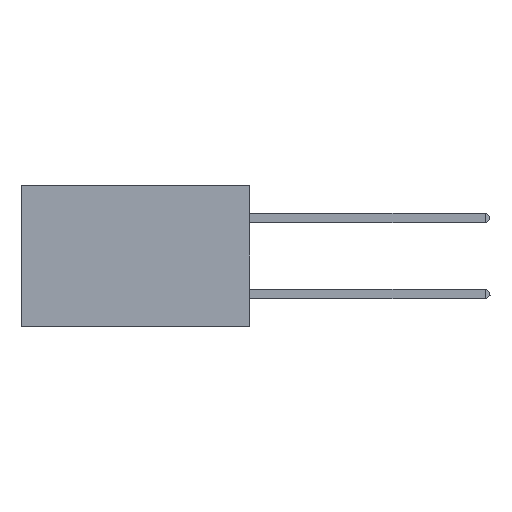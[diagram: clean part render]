
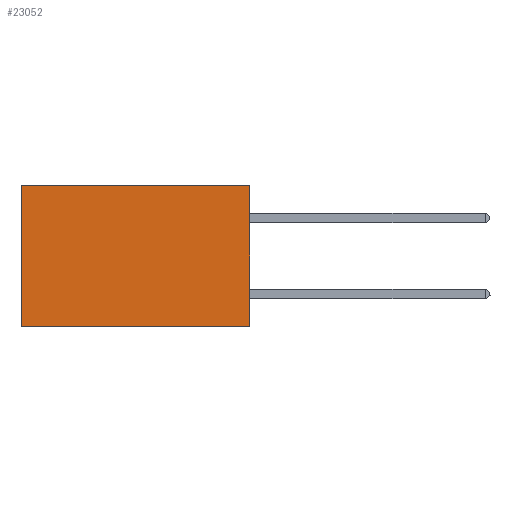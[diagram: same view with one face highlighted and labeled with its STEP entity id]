
A CAD part, left-side view. The second image highlights one B-rep face of the part: STEP entity #23052.
In plain terms, the highlighted planar face has unit normal (-1, 0, 0).
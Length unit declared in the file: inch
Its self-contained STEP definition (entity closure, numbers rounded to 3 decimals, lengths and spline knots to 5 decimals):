
#237 = FACE_OUTER_BOUND ( 'NONE', #17870, .T. ) ;
#645 = CARTESIAN_POINT ( 'NONE',  ( 0.2875, 0., 0. ) ) ;
#1793 = EDGE_CURVE ( 'NONE', #4694, #19247, #15864, .T. ) ;
#3028 = DIRECTION ( 'NONE',  ( 0., 0., -1. ) ) ;
#3229 = DIRECTION ( 'NONE',  ( 0., 0., -1. ) ) ;
#4694 = VERTEX_POINT ( 'NONE', #20214 ) ;
#5018 = EDGE_CURVE ( 'NONE', #10851, #4694, #14212, .T. ) ;
#5199 = DIRECTION ( 'NONE',  ( 0., 1., 0. ) ) ;
#7145 = EDGE_CURVE ( 'NONE', #10851, #10765, #13715, .T. ) ;
#8940 = DIRECTION ( 'NONE',  ( 0., 1., 0. ) ) ;
#9020 = ORIENTED_EDGE ( 'NONE', *, *, #13506, .F. ) ;
#9150 = ORIENTED_EDGE ( 'NONE', *, *, #7145, .F. ) ;
#10765 = VERTEX_POINT ( 'NONE', #15515 ) ;
#10851 = VERTEX_POINT ( 'NONE', #16892 ) ;
#13084 = CARTESIAN_POINT ( 'NONE',  ( 0.2875, 0., -0.37 ) ) ;
#13506 = EDGE_CURVE ( 'NONE', #10765, #19247, #14063, .T. ) ;
#13715 = LINE ( 'NONE', #645, #14093 ) ;
#14063 = LINE ( 'NONE', #13084, #25969 ) ;
#14093 = VECTOR ( 'NONE', #3028, 39.37008 ) ;
#14212 = LINE ( 'NONE', #28877, #22821 ) ;
#14662 = CARTESIAN_POINT ( 'NONE',  ( 0.2875, 0., 0. ) ) ;
#15515 = CARTESIAN_POINT ( 'NONE',  ( 0.2875, 0., -0.37 ) ) ;
#15864 = LINE ( 'NONE', #17469, #30058 ) ;
#16892 = CARTESIAN_POINT ( 'NONE',  ( 0.2875, 0., 0. ) ) ;
#17469 = CARTESIAN_POINT ( 'NONE',  ( 0.2875, 0.6, 0. ) ) ;
#17870 = EDGE_LOOP ( 'NONE', ( #21938, #9020, #9150, #18020 ) ) ;
#18020 = ORIENTED_EDGE ( 'NONE', *, *, #5018, .T. ) ;
#19247 = VERTEX_POINT ( 'NONE', #23455 ) ;
#20214 = CARTESIAN_POINT ( 'NONE',  ( 0.2875, 0.6, 0. ) ) ;
#21743 = PLANE ( 'NONE',  #28829 ) ;
#21938 = ORIENTED_EDGE ( 'NONE', *, *, #1793, .T. ) ;
#22821 = VECTOR ( 'NONE', #5199, 39.37008 ) ;
#23052 = ADVANCED_FACE ( 'NONE', ( #237 ), #21743, .F. ) ;
#23455 = CARTESIAN_POINT ( 'NONE',  ( 0.2875, 0.6, -0.37 ) ) ;
#25969 = VECTOR ( 'NONE', #8940, 39.37008 ) ;
#26452 = DIRECTION ( 'NONE',  ( 0., 0., -1. ) ) ;
#28829 = AXIS2_PLACEMENT_3D ( 'NONE', #14662, #29065, #26452 ) ;
#28877 = CARTESIAN_POINT ( 'NONE',  ( 0.2875, 0., 0. ) ) ;
#29065 = DIRECTION ( 'NONE',  ( 1., 0., 0. ) ) ;
#30058 = VECTOR ( 'NONE', #3229, 39.37008 ) ;
